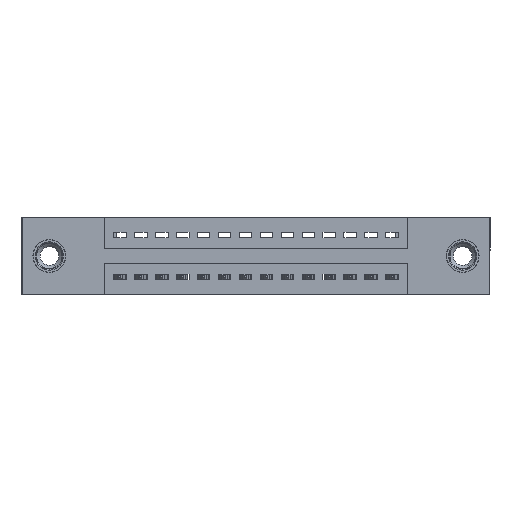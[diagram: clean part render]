
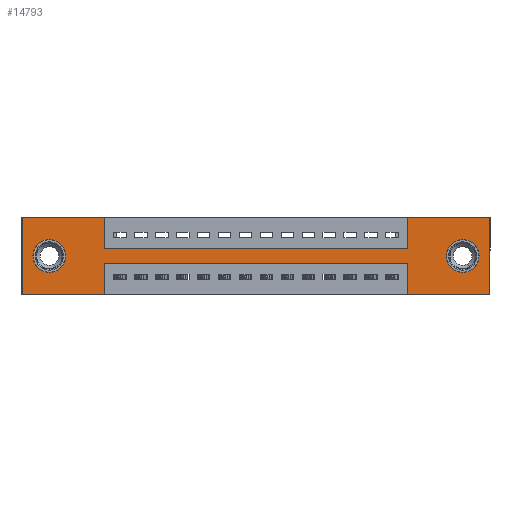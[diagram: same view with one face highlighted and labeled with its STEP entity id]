
A CAD part, front view. The second image highlights one B-rep face of the part: STEP entity #14793.
In plain terms, the highlighted planar face has unit normal (0, -1, 0).
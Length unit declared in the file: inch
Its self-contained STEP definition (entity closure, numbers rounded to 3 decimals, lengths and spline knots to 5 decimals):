
#130 = EDGE_CURVE ( 'NONE', #4794, #7486, #14220, .T. ) ;
#231 = CARTESIAN_POINT ( 'NONE',  ( 0.13, 0., -0.263 ) ) ;
#402 = CIRCLE ( 'NONE', #18330, 0.078 ) ;
#498 = EDGE_CURVE ( 'NONE', #10665, #4794, #7265, .T. ) ;
#573 = CARTESIAN_POINT ( 'NONE',  ( 0., 0., -0.37 ) ) ;
#781 = ORIENTED_EDGE ( 'NONE', *, *, #498, .F. ) ;
#952 = EDGE_CURVE ( 'NONE', #6716, #1665, #16957, .T. ) ;
#1273 = DIRECTION ( 'NONE',  ( 0., 0., -1. ) ) ;
#1584 = EDGE_CURVE ( 'NONE', #3624, #6716, #17871, .T. ) ;
#1655 = CIRCLE ( 'NONE', #15608, 0.078 ) ;
#1665 = VERTEX_POINT ( 'NONE', #6191 ) ;
#2029 = ORIENTED_EDGE ( 'NONE', *, *, #15205, .T. ) ;
#2319 = EDGE_CURVE ( 'NONE', #6546, #13896, #1655, .T. ) ;
#2656 = CARTESIAN_POINT ( 'NONE',  ( 0.13, 0., -0.185 ) ) ;
#2716 = CIRCLE ( 'NONE', #6600, 0.078 ) ;
#2733 = ORIENTED_EDGE ( 'NONE', *, *, #17627, .F. ) ;
#2761 = CARTESIAN_POINT ( 'NONE',  ( 0., 0., -0.37 ) ) ;
#2767 = VERTEX_POINT ( 'NONE', #9573 ) ;
#2838 = ORIENTED_EDGE ( 'NONE', *, *, #10027, .F. ) ;
#2849 = VECTOR ( 'NONE', #10859, 39.37008 ) ;
#3147 = CARTESIAN_POINT ( 'NONE',  ( 0.13, 0., -0.107 ) ) ;
#3198 = DIRECTION ( 'NONE',  ( -1., 0., 0. ) ) ;
#3444 = VERTEX_POINT ( 'NONE', #231 ) ;
#3624 = VERTEX_POINT ( 'NONE', #5262 ) ;
#3849 = CARTESIAN_POINT ( 'NONE',  ( 0.3925, 0., -0.15 ) ) ;
#3910 = EDGE_CURVE ( 'NONE', #10579, #6967, #17486, .T. ) ;
#4003 = DIRECTION ( 'NONE',  ( 0., 1., 0. ) ) ;
#4233 = CARTESIAN_POINT ( 'NONE',  ( 0., 0., 0. ) ) ;
#4443 = VERTEX_POINT ( 'NONE', #17525 ) ;
#4476 = LINE ( 'NONE', #3849, #17675 ) ;
#4628 = EDGE_CURVE ( 'NONE', #10166, #3444, #402, .T. ) ;
#4717 = AXIS2_PLACEMENT_3D ( 'NONE', #18928, #7231, #16034 ) ;
#4794 = VERTEX_POINT ( 'NONE', #6669 ) ;
#5207 = LINE ( 'NONE', #9215, #6369 ) ;
#5262 = CARTESIAN_POINT ( 'NONE',  ( 2.235, 0., 0. ) ) ;
#5459 = ORIENTED_EDGE ( 'NONE', *, *, #130, .F. ) ;
#5875 = VECTOR ( 'NONE', #16381, 39.37008 ) ;
#6191 = CARTESIAN_POINT ( 'NONE',  ( 1.8425, 0., -0.37 ) ) ;
#6369 = VECTOR ( 'NONE', #3198, 39.37008 ) ;
#6546 = VERTEX_POINT ( 'NONE', #15796 ) ;
#6600 = AXIS2_PLACEMENT_3D ( 'NONE', #14467, #4003, #7160 ) ;
#6669 = CARTESIAN_POINT ( 'NONE',  ( 0.3925, 0., -0.37 ) ) ;
#6692 = CARTESIAN_POINT ( 'NONE',  ( 0.3925, 0., 0. ) ) ;
#6716 = VERTEX_POINT ( 'NONE', #10081 ) ;
#6967 = VERTEX_POINT ( 'NONE', #10648 ) ;
#7160 = DIRECTION ( 'NONE',  ( 0., 0., 1. ) ) ;
#7185 = LINE ( 'NONE', #11148, #18505 ) ;
#7231 = DIRECTION ( 'NONE',  ( 0., 1., 0. ) ) ;
#7244 = VECTOR ( 'NONE', #17118, 39.37008 ) ;
#7265 = LINE ( 'NONE', #7458, #5875 ) ;
#7458 = CARTESIAN_POINT ( 'NONE',  ( 0.3925, 0., -0.37 ) ) ;
#7486 = VERTEX_POINT ( 'NONE', #11194 ) ;
#7542 = VERTEX_POINT ( 'NONE', #9697 ) ;
#7956 = VECTOR ( 'NONE', #17502, 39.37008 ) ;
#7964 = ORIENTED_EDGE ( 'NONE', *, *, #10901, .F. ) ;
#8022 = CIRCLE ( 'NONE', #4717, 0.078 ) ;
#8318 = LINE ( 'NONE', #12960, #13651 ) ;
#8432 = DIRECTION ( 'NONE',  ( 0., 0., 1. ) ) ;
#8445 = VECTOR ( 'NONE', #14715, 39.37008 ) ;
#8611 = DIRECTION ( 'NONE',  ( -1., 0., 0. ) ) ;
#9215 = CARTESIAN_POINT ( 'NONE',  ( 0.3925, 0., -0.22 ) ) ;
#9372 = EDGE_LOOP ( 'NONE', ( #18278, #15827 ) ) ;
#9538 = ORIENTED_EDGE ( 'NONE', *, *, #1584, .F. ) ;
#9573 = CARTESIAN_POINT ( 'NONE',  ( 1.8425, 0., 0. ) ) ;
#9596 = EDGE_CURVE ( 'NONE', #2767, #3624, #13319, .T. ) ;
#9654 = DIRECTION ( 'NONE',  ( 0., 0., -1. ) ) ;
#9697 = CARTESIAN_POINT ( 'NONE',  ( 0.3925, 0., -0.15 ) ) ;
#9804 = LINE ( 'NONE', #4233, #7956 ) ;
#10027 = EDGE_CURVE ( 'NONE', #7486, #10579, #9804, .T. ) ;
#10081 = CARTESIAN_POINT ( 'NONE',  ( 2.235, 0., -0.37 ) ) ;
#10166 = VERTEX_POINT ( 'NONE', #3147 ) ;
#10274 = VECTOR ( 'NONE', #8611, 39.37008 ) ;
#10427 = ORIENTED_EDGE ( 'NONE', *, *, #13389, .F. ) ;
#10579 = VERTEX_POINT ( 'NONE', #11094 ) ;
#10648 = CARTESIAN_POINT ( 'NONE',  ( 0.3925, 0., 0. ) ) ;
#10665 = VERTEX_POINT ( 'NONE', #17839 ) ;
#10859 = DIRECTION ( 'NONE',  ( -1., 0., 0. ) ) ;
#10901 = EDGE_CURVE ( 'NONE', #7542, #15571, #4476, .T. ) ;
#11094 = CARTESIAN_POINT ( 'NONE',  ( 0., 0., 0. ) ) ;
#11148 = CARTESIAN_POINT ( 'NONE',  ( 1.8425, 0., -0.37 ) ) ;
#11158 = LINE ( 'NONE', #6692, #7244 ) ;
#11194 = CARTESIAN_POINT ( 'NONE',  ( 0., 0., -0.37 ) ) ;
#11227 = EDGE_LOOP ( 'NONE', ( #2029, #18496 ) ) ;
#11476 = ORIENTED_EDGE ( 'NONE', *, *, #952, .F. ) ;
#11886 = ORIENTED_EDGE ( 'NONE', *, *, #18869, .F. ) ;
#12384 = CARTESIAN_POINT ( 'NONE',  ( 2.105, 0., -0.107 ) ) ;
#12848 = VECTOR ( 'NONE', #13607, 39.37008 ) ;
#12878 = DIRECTION ( 'NONE',  ( 1., 0., 0. ) ) ;
#12960 = CARTESIAN_POINT ( 'NONE',  ( 1.8425, 0., 0. ) ) ;
#13187 = EDGE_CURVE ( 'NONE', #15571, #2767, #8318, .T. ) ;
#13319 = LINE ( 'NONE', #18183, #12848 ) ;
#13337 = CARTESIAN_POINT ( 'NONE',  ( 0., 0., 0. ) ) ;
#13389 = EDGE_CURVE ( 'NONE', #1665, #4443, #7185, .T. ) ;
#13396 = AXIS2_PLACEMENT_3D ( 'NONE', #16051, #14421, #1273 ) ;
#13607 = DIRECTION ( 'NONE',  ( 1., 0., 0. ) ) ;
#13651 = VECTOR ( 'NONE', #8432, 39.37008 ) ;
#13896 = VERTEX_POINT ( 'NONE', #12384 ) ;
#13929 = VECTOR ( 'NONE', #9654, 39.37008 ) ;
#13948 = DIRECTION ( 'NONE',  ( 0., 0., 1. ) ) ;
#14220 = LINE ( 'NONE', #2761, #10274 ) ;
#14421 = DIRECTION ( 'NONE',  ( 0., -1., 0. ) ) ;
#14467 = CARTESIAN_POINT ( 'NONE',  ( 0.13, 0., -0.185 ) ) ;
#14715 = DIRECTION ( 'NONE',  ( 1., 0., 0. ) ) ;
#14776 = FACE_BOUND ( 'NONE', #9372, .T. ) ;
#14793 = ADVANCED_FACE ( 'NONE', ( #18677, #14776, #15694 ), #17226, .T. ) ;
#15205 = EDGE_CURVE ( 'NONE', #13896, #6546, #8022, .T. ) ;
#15571 = VERTEX_POINT ( 'NONE', #16532 ) ;
#15580 = DIRECTION ( 'NONE',  ( 0., 1., 0. ) ) ;
#15608 = AXIS2_PLACEMENT_3D ( 'NONE', #18403, #15580, #18534 ) ;
#15680 = EDGE_LOOP ( 'NONE', ( #781, #2733, #10427, #11476, #9538, #17697, #18305, #7964, #11886, #18868, #2838, #5459 ) ) ;
#15694 = FACE_OUTER_BOUND ( 'NONE', #15680, .T. ) ;
#15796 = CARTESIAN_POINT ( 'NONE',  ( 2.105, 0., -0.263 ) ) ;
#15827 = ORIENTED_EDGE ( 'NONE', *, *, #16921, .T. ) ;
#16034 = DIRECTION ( 'NONE',  ( 0., 0., -1. ) ) ;
#16051 = CARTESIAN_POINT ( 'NONE',  ( 0., 0., -0.37 ) ) ;
#16381 = DIRECTION ( 'NONE',  ( 0., 0., -1. ) ) ;
#16532 = CARTESIAN_POINT ( 'NONE',  ( 1.8425, 0., -0.15 ) ) ;
#16921 = EDGE_CURVE ( 'NONE', #3444, #10166, #2716, .T. ) ;
#16957 = LINE ( 'NONE', #573, #2849 ) ;
#17118 = DIRECTION ( 'NONE',  ( 0., 0., -1. ) ) ;
#17132 = DIRECTION ( 'NONE',  ( 0., 0., 1. ) ) ;
#17226 = PLANE ( 'NONE',  #13396 ) ;
#17486 = LINE ( 'NONE', #13337, #8445 ) ;
#17502 = DIRECTION ( 'NONE',  ( 0., 0., 1. ) ) ;
#17525 = CARTESIAN_POINT ( 'NONE',  ( 1.8425, 0., -0.22 ) ) ;
#17627 = EDGE_CURVE ( 'NONE', #4443, #10665, #5207, .T. ) ;
#17675 = VECTOR ( 'NONE', #12878, 39.37008 ) ;
#17697 = ORIENTED_EDGE ( 'NONE', *, *, #9596, .F. ) ;
#17839 = CARTESIAN_POINT ( 'NONE',  ( 0.3925, 0., -0.22 ) ) ;
#17871 = LINE ( 'NONE', #18529, #13929 ) ;
#18183 = CARTESIAN_POINT ( 'NONE',  ( 0., 0., 0. ) ) ;
#18278 = ORIENTED_EDGE ( 'NONE', *, *, #4628, .T. ) ;
#18305 = ORIENTED_EDGE ( 'NONE', *, *, #13187, .F. ) ;
#18330 = AXIS2_PLACEMENT_3D ( 'NONE', #2656, #18459, #13948 ) ;
#18403 = CARTESIAN_POINT ( 'NONE',  ( 2.105, 0., -0.185 ) ) ;
#18459 = DIRECTION ( 'NONE',  ( 0., 1., 0. ) ) ;
#18496 = ORIENTED_EDGE ( 'NONE', *, *, #2319, .T. ) ;
#18505 = VECTOR ( 'NONE', #17132, 39.37008 ) ;
#18529 = CARTESIAN_POINT ( 'NONE',  ( 2.235, 0., 0. ) ) ;
#18534 = DIRECTION ( 'NONE',  ( 0., 0., -1. ) ) ;
#18677 = FACE_BOUND ( 'NONE', #11227, .T. ) ;
#18868 = ORIENTED_EDGE ( 'NONE', *, *, #3910, .F. ) ;
#18869 = EDGE_CURVE ( 'NONE', #6967, #7542, #11158, .T. ) ;
#18928 = CARTESIAN_POINT ( 'NONE',  ( 2.105, 0., -0.185 ) ) ;
